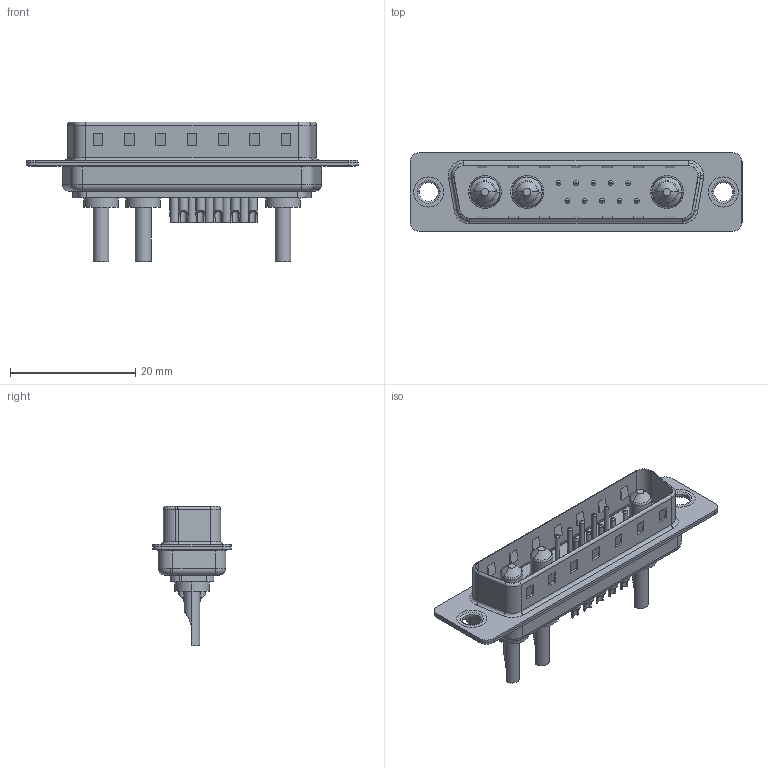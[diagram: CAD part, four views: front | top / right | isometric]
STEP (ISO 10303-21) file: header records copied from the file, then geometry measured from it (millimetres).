
FILE_DESCRIPTION (( 'STEP AP203' ), '1' );
FILE_NAME ('627-13W3222-1N1.STEP', '2019-05-26T11:44:42', ( '' ), ( '' ), 'SwSTEP 2.0', 'SolidWorks 2016', '' );
FILE_SCHEMA (( 'CONFIG_CONTROL_DESIGN' ));
Length unit declared in the file: millimetre
Products named in the file (8): Power Pin_10A SC; 627Combo Contact Row 1_22; 627Combo Contact Row 2_22; 627-13W3222-1N1; 627Combo Housing_13W3; 627Combo Shell Rear_25 Contacts; 627Combo Shell Front_25 Contacts; 627Combo Thru Hole Rivet
Assembly tree (18 placements, depth 2):
  627-13W3222-1N1
    627Combo Housing_13W3
    627Combo Shell Rear_25 Contacts
    627Combo Shell Front_25 Contacts
    627Combo Thru Hole Rivet  x2
    Power Pin_10A SC  x3
    627Combo Contact Row 1_22  x5
    627Combo Contact Row 2_22  x5
Bounding box: 53 x 12.6 x 22.3 mm (x, y, z)
Volume: 2854.2 mm3; surface area: 6826.4 mm2
Topology: 21 solids, 21 shells, 855 faces, 2012 edges, 1233 vertices
Faces by surface type: cylinder 347, plane 297, torus 164, cone 41, bspline 6
Entity records: 16755 total; most frequent: DIRECTION 2852, CARTESIAN_POINT 2843, ORIENTED_EDGE 2524, EDGE_CURVE 1262, AXIS2_PLACEMENT_3D 1089, VERTEX_POINT 795, VECTOR 674, LINE 674
